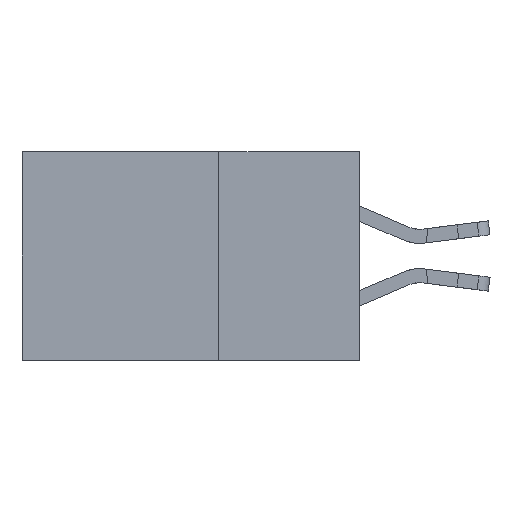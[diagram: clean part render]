
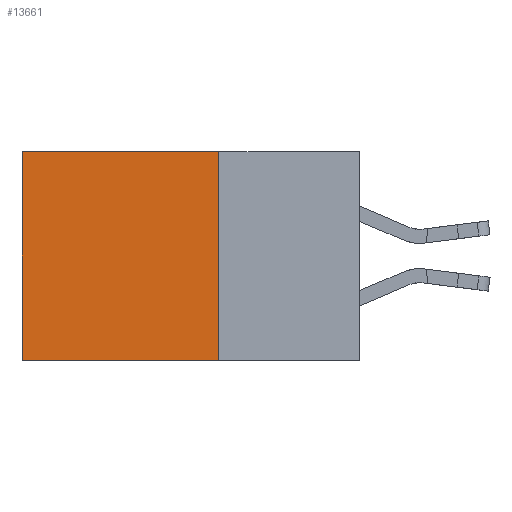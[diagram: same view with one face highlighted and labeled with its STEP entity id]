
A CAD part, left-side view. The second image highlights one B-rep face of the part: STEP entity #13661.
In plain terms, the highlighted planar face has unit normal (-1, 0, 0).
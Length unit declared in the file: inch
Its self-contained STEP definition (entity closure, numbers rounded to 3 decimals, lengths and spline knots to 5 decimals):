
#258 = CARTESIAN_POINT ( 'NONE',  ( 0.2875, 0.25, 0. ) ) ;
#368 = VERTEX_POINT ( 'NONE', #15387 ) ;
#484 = LINE ( 'NONE', #4615, #8936 ) ;
#1348 = ORIENTED_EDGE ( 'NONE', *, *, #8881, .T. ) ;
#1413 = CARTESIAN_POINT ( 'NONE',  ( 0.2875, 0.25, 0. ) ) ;
#1708 = LINE ( 'NONE', #8044, #13923 ) ;
#1902 = CARTESIAN_POINT ( 'NONE',  ( 0.2875, 0.25, 0. ) ) ;
#2415 = FACE_OUTER_BOUND ( 'NONE', #9780, .T. ) ;
#3021 = EDGE_CURVE ( 'NONE', #9668, #3548, #5839, .T. ) ;
#3175 = VECTOR ( 'NONE', #16599, 39.37008 ) ;
#3548 = VERTEX_POINT ( 'NONE', #15940 ) ;
#3582 = DIRECTION ( 'NONE',  ( 0., 0., -1. ) ) ;
#4615 = CARTESIAN_POINT ( 'NONE',  ( 0.2875, 0.25, -0.37 ) ) ;
#5436 = CARTESIAN_POINT ( 'NONE',  ( 0.2875, 0.6, 0. ) ) ;
#5839 = LINE ( 'NONE', #5436, #3175 ) ;
#7564 = ORIENTED_EDGE ( 'NONE', *, *, #3021, .T. ) ;
#8044 = CARTESIAN_POINT ( 'NONE',  ( 0.2875, 0.25, 0. ) ) ;
#8881 = EDGE_CURVE ( 'NONE', #18173, #9668, #9552, .T. ) ;
#8936 = VECTOR ( 'NONE', #13237, 39.37008 ) ;
#9552 = LINE ( 'NONE', #258, #14645 ) ;
#9668 = VERTEX_POINT ( 'NONE', #15942 ) ;
#9780 = EDGE_LOOP ( 'NONE', ( #7564, #18042, #16643, #1348 ) ) ;
#10489 = EDGE_CURVE ( 'NONE', #18173, #368, #1708, .T. ) ;
#10853 = EDGE_CURVE ( 'NONE', #368, #3548, #484, .T. ) ;
#11753 = DIRECTION ( 'NONE',  ( 0., 1., 0. ) ) ;
#11768 = PLANE ( 'NONE',  #18133 ) ;
#13076 = DIRECTION ( 'NONE',  ( 1., 0., 0. ) ) ;
#13203 = DIRECTION ( 'NONE',  ( 0., 0., -1. ) ) ;
#13237 = DIRECTION ( 'NONE',  ( 0., 1., 0. ) ) ;
#13661 = ADVANCED_FACE ( 'NONE', ( #2415 ), #11768, .F. ) ;
#13923 = VECTOR ( 'NONE', #3582, 39.37008 ) ;
#14645 = VECTOR ( 'NONE', #11753, 39.37008 ) ;
#15387 = CARTESIAN_POINT ( 'NONE',  ( 0.2875, 0.25, -0.37 ) ) ;
#15940 = CARTESIAN_POINT ( 'NONE',  ( 0.2875, 0.6, -0.37 ) ) ;
#15942 = CARTESIAN_POINT ( 'NONE',  ( 0.2875, 0.6, 0. ) ) ;
#16599 = DIRECTION ( 'NONE',  ( 0., 0., -1. ) ) ;
#16643 = ORIENTED_EDGE ( 'NONE', *, *, #10489, .F. ) ;
#18042 = ORIENTED_EDGE ( 'NONE', *, *, #10853, .F. ) ;
#18133 = AXIS2_PLACEMENT_3D ( 'NONE', #1902, #13076, #13203 ) ;
#18173 = VERTEX_POINT ( 'NONE', #1413 ) ;
